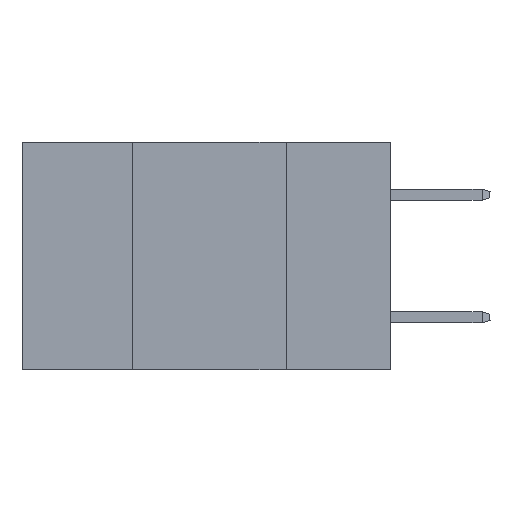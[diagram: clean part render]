
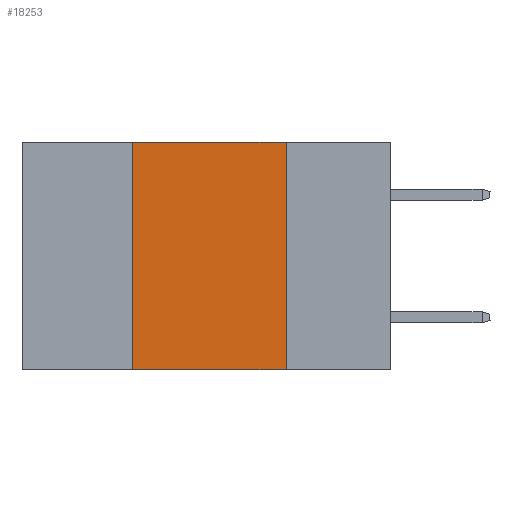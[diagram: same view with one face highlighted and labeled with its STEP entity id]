
A CAD part, left-side view. The second image highlights one B-rep face of the part: STEP entity #18253.
In plain terms, the highlighted planar face has unit normal (-1, 0, 0).
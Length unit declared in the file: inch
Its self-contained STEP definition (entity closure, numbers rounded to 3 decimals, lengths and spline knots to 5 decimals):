
#109 = VECTOR ( 'NONE', #25341, 39.37008 ) ;
#318 = ORIENTED_EDGE ( 'NONE', *, *, #18765, .F. ) ;
#1516 = AXIS2_PLACEMENT_3D ( 'NONE', #15626, #21717, #9566 ) ;
#1664 = LINE ( 'NONE', #21247, #16870 ) ;
#1992 = FACE_OUTER_BOUND ( 'NONE', #13819, .T. ) ;
#2172 = ORIENTED_EDGE ( 'NONE', *, *, #4217, .T. ) ;
#2469 = VERTEX_POINT ( 'NONE', #23697 ) ;
#3124 = ORIENTED_EDGE ( 'NONE', *, *, #10328, .F. ) ;
#4217 = EDGE_CURVE ( 'NONE', #2469, #7857, #1664, .T. ) ;
#4425 = LINE ( 'NONE', #11196, #109 ) ;
#7106 = DIRECTION ( 'NONE',  ( 0., -1., 0. ) ) ;
#7489 = PLANE ( 'NONE',  #1516 ) ;
#7857 = VERTEX_POINT ( 'NONE', #17479 ) ;
#9566 = DIRECTION ( 'NONE',  ( 0., 0., -1. ) ) ;
#10328 = EDGE_CURVE ( 'NONE', #2469, #12636, #4425, .T. ) ;
#11196 = CARTESIAN_POINT ( 'NONE',  ( 0., 0.42, 0. ) ) ;
#11296 = VECTOR ( 'NONE', #12999, 39.37008 ) ;
#12194 = ORIENTED_EDGE ( 'NONE', *, *, #20673, .F. ) ;
#12636 = VERTEX_POINT ( 'NONE', #14524 ) ;
#12999 = DIRECTION ( 'NONE',  ( 0., 0., -1. ) ) ;
#13819 = EDGE_LOOP ( 'NONE', ( #12194, #318, #3124, #2172 ) ) ;
#14524 = CARTESIAN_POINT ( 'NONE',  ( 0., 0.42, 0. ) ) ;
#15626 = CARTESIAN_POINT ( 'NONE',  ( 0., 0.6, 0. ) ) ;
#15783 = CARTESIAN_POINT ( 'NONE',  ( 0., 0.17, 0. ) ) ;
#16127 = VERTEX_POINT ( 'NONE', #15783 ) ;
#16870 = VECTOR ( 'NONE', #17109, 39.37008 ) ;
#17109 = DIRECTION ( 'NONE',  ( 0., -1., 0. ) ) ;
#17479 = CARTESIAN_POINT ( 'NONE',  ( 0., 0.17, -0.37 ) ) ;
#18253 = ADVANCED_FACE ( 'NONE', ( #1992 ), #7489, .F. ) ;
#18765 = EDGE_CURVE ( 'NONE', #12636, #16127, #23138, .T. ) ;
#20673 = EDGE_CURVE ( 'NONE', #16127, #7857, #22712, .T. ) ;
#21247 = CARTESIAN_POINT ( 'NONE',  ( 0., 0.6, -0.37 ) ) ;
#21340 = CARTESIAN_POINT ( 'NONE',  ( 0., 0.6, 0. ) ) ;
#21717 = DIRECTION ( 'NONE',  ( 1., 0., 0. ) ) ;
#22712 = LINE ( 'NONE', #23185, #11296 ) ;
#23138 = LINE ( 'NONE', #21340, #25987 ) ;
#23185 = CARTESIAN_POINT ( 'NONE',  ( 0., 0.17, 0. ) ) ;
#23697 = CARTESIAN_POINT ( 'NONE',  ( 0., 0.42, -0.37 ) ) ;
#25341 = DIRECTION ( 'NONE',  ( 0., 0., 1. ) ) ;
#25987 = VECTOR ( 'NONE', #7106, 39.37008 ) ;
